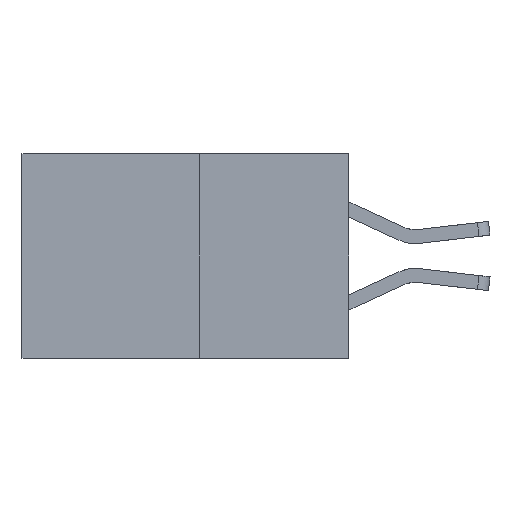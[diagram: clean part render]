
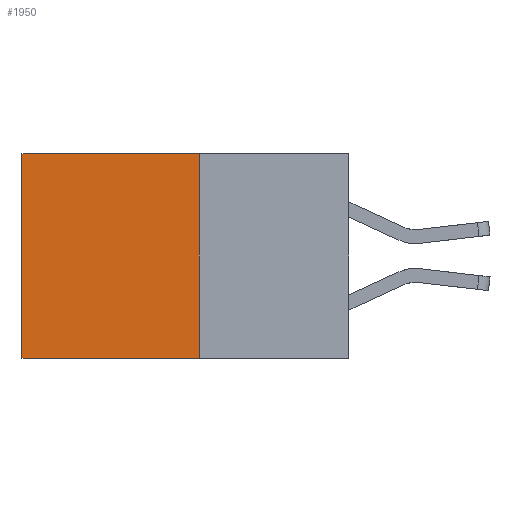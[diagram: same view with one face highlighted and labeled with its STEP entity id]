
A CAD part, left-side view. The second image highlights one B-rep face of the part: STEP entity #1950.
In plain terms, the highlighted planar face has unit normal (-1, 0, 0).
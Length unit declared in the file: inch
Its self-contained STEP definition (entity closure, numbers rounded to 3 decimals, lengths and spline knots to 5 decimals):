
#650 = VECTOR ( 'NONE', #6759, 39.37008 ) ;
#947 = CARTESIAN_POINT ( 'NONE',  ( 0.277, 0.27, -0.37 ) ) ;
#1454 = LINE ( 'NONE', #4001, #8703 ) ;
#1950 = ADVANCED_FACE ( 'NONE', ( #4358 ), #4272, .F. ) ;
#2074 = ORIENTED_EDGE ( 'NONE', *, *, #5724, .T. ) ;
#2180 = CARTESIAN_POINT ( 'NONE',  ( 0.277, 0.59, 0. ) ) ;
#2470 = VERTEX_POINT ( 'NONE', #2180 ) ;
#2651 = ORIENTED_EDGE ( 'NONE', *, *, #4416, .F. ) ;
#2774 = ORIENTED_EDGE ( 'NONE', *, *, #4475, .F. ) ;
#2976 = AXIS2_PLACEMENT_3D ( 'NONE', #4265, #7718, #5366 ) ;
#3065 = VECTOR ( 'NONE', #8558, 39.37008 ) ;
#3253 = LINE ( 'NONE', #6788, #650 ) ;
#3598 = DIRECTION ( 'NONE',  ( 0., 1., 0. ) ) ;
#4001 = CARTESIAN_POINT ( 'NONE',  ( 0.277, 0.27, -0.37 ) ) ;
#4005 = VECTOR ( 'NONE', #4414, 39.37008 ) ;
#4265 = CARTESIAN_POINT ( 'NONE',  ( 0.277, 0.27, -0.37 ) ) ;
#4272 = PLANE ( 'NONE',  #2976 ) ;
#4358 = FACE_OUTER_BOUND ( 'NONE', #6627, .T. ) ;
#4414 = DIRECTION ( 'NONE',  ( 0., 0., -1. ) ) ;
#4416 = EDGE_CURVE ( 'NONE', #5659, #7862, #5799, .T. ) ;
#4475 = EDGE_CURVE ( 'NONE', #7862, #6521, #1454, .T. ) ;
#5366 = DIRECTION ( 'NONE',  ( 0., 0., -1. ) ) ;
#5534 = CARTESIAN_POINT ( 'NONE',  ( 0.277, 0.59, -0.37 ) ) ;
#5598 = CARTESIAN_POINT ( 'NONE',  ( 0.277, 0.27, -0.37 ) ) ;
#5659 = VERTEX_POINT ( 'NONE', #5951 ) ;
#5724 = EDGE_CURVE ( 'NONE', #5659, #2470, #3253, .T. ) ;
#5799 = LINE ( 'NONE', #5598, #4005 ) ;
#5951 = CARTESIAN_POINT ( 'NONE',  ( 0.277, 0.27, 0. ) ) ;
#6004 = ORIENTED_EDGE ( 'NONE', *, *, #6995, .T. ) ;
#6521 = VERTEX_POINT ( 'NONE', #5534 ) ;
#6627 = EDGE_LOOP ( 'NONE', ( #6004, #2774, #2651, #2074 ) ) ;
#6759 = DIRECTION ( 'NONE',  ( 0., 1., 0. ) ) ;
#6788 = CARTESIAN_POINT ( 'NONE',  ( 0.277, 0.27, 0. ) ) ;
#6995 = EDGE_CURVE ( 'NONE', #2470, #6521, #8446, .T. ) ;
#7718 = DIRECTION ( 'NONE',  ( 1., 0., 0. ) ) ;
#7854 = CARTESIAN_POINT ( 'NONE',  ( 0.277, 0.59, -0.37 ) ) ;
#7862 = VERTEX_POINT ( 'NONE', #947 ) ;
#8446 = LINE ( 'NONE', #7854, #3065 ) ;
#8558 = DIRECTION ( 'NONE',  ( 0., 0., -1. ) ) ;
#8703 = VECTOR ( 'NONE', #3598, 39.37008 ) ;
